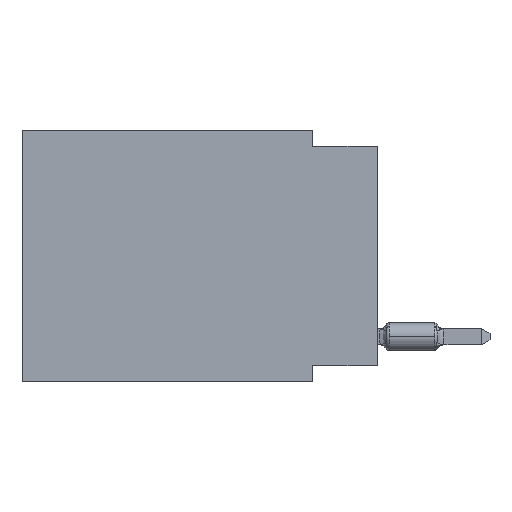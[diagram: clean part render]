
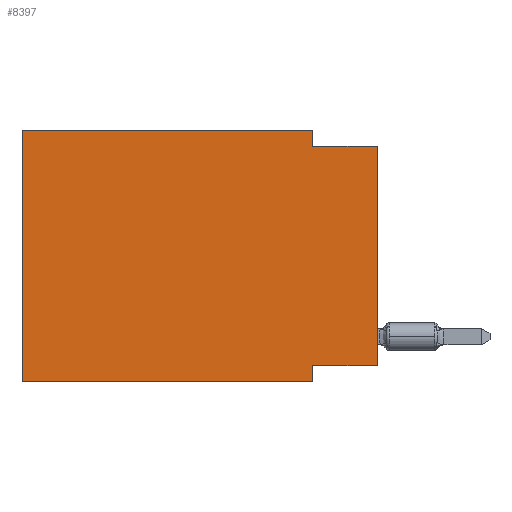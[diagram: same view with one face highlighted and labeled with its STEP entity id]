
A CAD part, left-side view. The second image highlights one B-rep face of the part: STEP entity #8397.
In plain terms, the highlighted planar face has unit normal (-1, 0, 0).
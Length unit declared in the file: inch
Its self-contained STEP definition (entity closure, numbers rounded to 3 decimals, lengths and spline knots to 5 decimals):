
#618 = ORIENTED_EDGE ( 'NONE', *, *, #860, .F. ) ;
#821 = ORIENTED_EDGE ( 'NONE', *, *, #5790, .F. ) ;
#860 = EDGE_CURVE ( 'NONE', #10767, #10580, #11166, .T. ) ;
#1049 = VERTEX_POINT ( 'NONE', #5589 ) ;
#1361 = DIRECTION ( 'NONE',  ( 0., 0., 1. ) ) ;
#1573 = LINE ( 'NONE', #5271, #15114 ) ;
#1697 = AXIS2_PLACEMENT_3D ( 'NONE', #13831, #4213, #3040 ) ;
#2516 = CARTESIAN_POINT ( 'NONE',  ( 0., 0., 0. ) ) ;
#2611 = CARTESIAN_POINT ( 'NONE',  ( 0., 0.55, 0. ) ) ;
#2792 = EDGE_CURVE ( 'NONE', #9519, #6800, #13429, .T. ) ;
#2807 = CARTESIAN_POINT ( 'NONE',  ( 0., 0.1, -0.365 ) ) ;
#2872 = VECTOR ( 'NONE', #14626, 39.37008 ) ;
#3040 = DIRECTION ( 'NONE',  ( 0., 0., -1. ) ) ;
#3250 = CARTESIAN_POINT ( 'NONE',  ( 0., 0.1, 0. ) ) ;
#3480 = DIRECTION ( 'NONE',  ( 0., 0., -1. ) ) ;
#4012 = DIRECTION ( 'NONE',  ( 0., -1., 0. ) ) ;
#4211 = EDGE_CURVE ( 'NONE', #8217, #10767, #10957, .T. ) ;
#4213 = DIRECTION ( 'NONE',  ( 1., 0., 0. ) ) ;
#4225 = CARTESIAN_POINT ( 'NONE',  ( 0., 0., -0.365 ) ) ;
#4306 = EDGE_CURVE ( 'NONE', #1049, #6433, #5359, .T. ) ;
#5242 = PLANE ( 'NONE',  #1697 ) ;
#5271 = CARTESIAN_POINT ( 'NONE',  ( 0., 0., -0.365 ) ) ;
#5359 = LINE ( 'NONE', #10239, #8303 ) ;
#5522 = ORIENTED_EDGE ( 'NONE', *, *, #2792, .F. ) ;
#5589 = CARTESIAN_POINT ( 'NONE',  ( 0., 0.1, -0.025 ) ) ;
#5692 = EDGE_CURVE ( 'NONE', #8217, #6800, #9839, .T. ) ;
#5790 = EDGE_CURVE ( 'NONE', #11760, #9519, #1573, .T. ) ;
#6215 = VECTOR ( 'NONE', #4012, 39.37008 ) ;
#6433 = VERTEX_POINT ( 'NONE', #9497 ) ;
#6796 = CARTESIAN_POINT ( 'NONE',  ( 0., 0.1, 0. ) ) ;
#6800 = VERTEX_POINT ( 'NONE', #11839 ) ;
#7331 = CARTESIAN_POINT ( 'NONE',  ( 0., 0.55, -0.39 ) ) ;
#7521 = ORIENTED_EDGE ( 'NONE', *, *, #5692, .T. ) ;
#8217 = VERTEX_POINT ( 'NONE', #13282 ) ;
#8303 = VECTOR ( 'NONE', #12858, 39.37008 ) ;
#8397 = ADVANCED_FACE ( 'NONE', ( #10120 ), #5242, .F. ) ;
#8649 = LINE ( 'NONE', #2516, #2872 ) ;
#9497 = CARTESIAN_POINT ( 'NONE',  ( 0., 0., -0.025 ) ) ;
#9519 = VERTEX_POINT ( 'NONE', #2807 ) ;
#9570 = ORIENTED_EDGE ( 'NONE', *, *, #14352, .T. ) ;
#9839 = LINE ( 'NONE', #7331, #14120 ) ;
#9905 = DIRECTION ( 'NONE',  ( 0., -1., 0. ) ) ;
#9990 = ORIENTED_EDGE ( 'NONE', *, *, #4211, .F. ) ;
#10120 = FACE_OUTER_BOUND ( 'NONE', #11809, .T. ) ;
#10239 = CARTESIAN_POINT ( 'NONE',  ( 0., 0., -0.025 ) ) ;
#10424 = VECTOR ( 'NONE', #14534, 39.37008 ) ;
#10550 = ORIENTED_EDGE ( 'NONE', *, *, #13892, .F. ) ;
#10580 = VERTEX_POINT ( 'NONE', #6796 ) ;
#10767 = VERTEX_POINT ( 'NONE', #14332 ) ;
#10957 = LINE ( 'NONE', #2611, #15551 ) ;
#11019 = DIRECTION ( 'NONE',  ( 0., 1., 0. ) ) ;
#11166 = LINE ( 'NONE', #13544, #6215 ) ;
#11760 = VERTEX_POINT ( 'NONE', #4225 ) ;
#11809 = EDGE_LOOP ( 'NONE', ( #9570, #12765, #10550, #618, #9990, #7521, #5522, #821 ) ) ;
#11839 = CARTESIAN_POINT ( 'NONE',  ( 0., 0.1, -0.39 ) ) ;
#12765 = ORIENTED_EDGE ( 'NONE', *, *, #4306, .F. ) ;
#12858 = DIRECTION ( 'NONE',  ( 0., -1., 0. ) ) ;
#13282 = CARTESIAN_POINT ( 'NONE',  ( 0., 0.55, -0.39 ) ) ;
#13429 = LINE ( 'NONE', #14458, #10424 ) ;
#13544 = CARTESIAN_POINT ( 'NONE',  ( 0., 0.55, 0. ) ) ;
#13831 = CARTESIAN_POINT ( 'NONE',  ( 0., 0.55, 0. ) ) ;
#13892 = EDGE_CURVE ( 'NONE', #10580, #1049, #14270, .T. ) ;
#14120 = VECTOR ( 'NONE', #9905, 39.37008 ) ;
#14183 = VECTOR ( 'NONE', #3480, 39.37008 ) ;
#14270 = LINE ( 'NONE', #3250, #14183 ) ;
#14332 = CARTESIAN_POINT ( 'NONE',  ( 0., 0.55, 0. ) ) ;
#14352 = EDGE_CURVE ( 'NONE', #11760, #6433, #8649, .T. ) ;
#14458 = CARTESIAN_POINT ( 'NONE',  ( 0., 0.1, -0.39 ) ) ;
#14534 = DIRECTION ( 'NONE',  ( 0., 0., -1. ) ) ;
#14626 = DIRECTION ( 'NONE',  ( 0., 0., 1. ) ) ;
#15114 = VECTOR ( 'NONE', #11019, 39.37008 ) ;
#15551 = VECTOR ( 'NONE', #1361, 39.37008 ) ;
